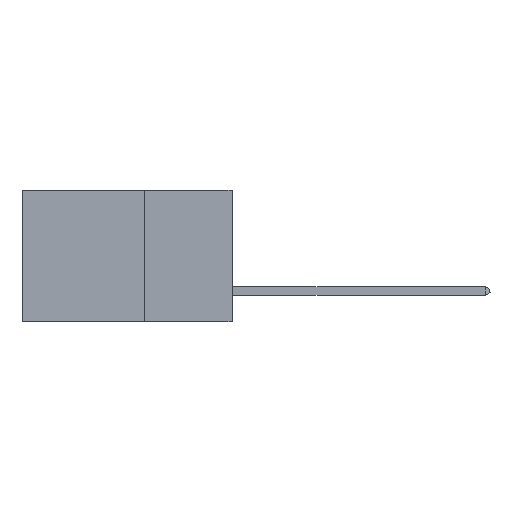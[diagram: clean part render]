
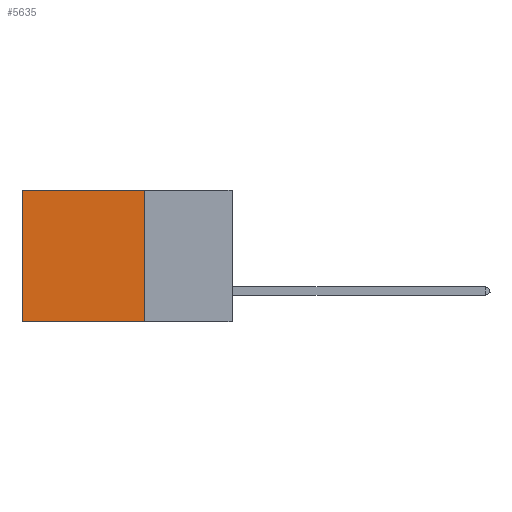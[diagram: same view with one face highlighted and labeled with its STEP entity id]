
A CAD part, left-side view. The second image highlights one B-rep face of the part: STEP entity #5635.
In plain terms, the highlighted planar face has unit normal (-1, 0, 0).
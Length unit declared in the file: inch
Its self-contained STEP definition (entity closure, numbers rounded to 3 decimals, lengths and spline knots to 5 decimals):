
#220 = CARTESIAN_POINT ( 'NONE',  ( 0.2875, 0.25, -0.375 ) ) ;
#1870 = ORIENTED_EDGE ( 'NONE', *, *, #9336, .T. ) ;
#2550 = VECTOR ( 'NONE', #4177, 39.37008 ) ;
#3336 = CARTESIAN_POINT ( 'NONE',  ( 0.2875, 0.6, -0.375 ) ) ;
#4177 = DIRECTION ( 'NONE',  ( 0., 1., 0. ) ) ;
#4750 = VECTOR ( 'NONE', #9437, 39.37008 ) ;
#4900 = LINE ( 'NONE', #13438, #2550 ) ;
#4920 = VECTOR ( 'NONE', #13117, 39.37008 ) ;
#5073 = VERTEX_POINT ( 'NONE', #14737 ) ;
#5245 = PLANE ( 'NONE',  #12274 ) ;
#5388 = EDGE_CURVE ( 'NONE', #11616, #7724, #6596, .T. ) ;
#5635 = ADVANCED_FACE ( 'NONE', ( #8237 ), #5245, .F. ) ;
#6083 = EDGE_CURVE ( 'NONE', #7082, #11616, #10578, .T. ) ;
#6199 = LINE ( 'NONE', #3336, #14768 ) ;
#6369 = DIRECTION ( 'NONE',  ( 0., 0., -1. ) ) ;
#6430 = CARTESIAN_POINT ( 'NONE',  ( 0.2875, 0.6, -0.375 ) ) ;
#6468 = CARTESIAN_POINT ( 'NONE',  ( 0.2875, 0.25, -0.375 ) ) ;
#6596 = LINE ( 'NONE', #9387, #4750 ) ;
#7082 = VERTEX_POINT ( 'NONE', #8293 ) ;
#7724 = VERTEX_POINT ( 'NONE', #6430 ) ;
#8237 = FACE_OUTER_BOUND ( 'NONE', #10676, .T. ) ;
#8293 = CARTESIAN_POINT ( 'NONE',  ( 0.2875, 0.25, 0. ) ) ;
#8301 = CARTESIAN_POINT ( 'NONE',  ( 0.2875, 0.25, -0.375 ) ) ;
#9336 = EDGE_CURVE ( 'NONE', #5073, #7724, #6199, .T. ) ;
#9387 = CARTESIAN_POINT ( 'NONE',  ( 0.2875, 0.25, -0.375 ) ) ;
#9437 = DIRECTION ( 'NONE',  ( 0., 1., 0. ) ) ;
#9484 = ORIENTED_EDGE ( 'NONE', *, *, #6083, .F. ) ;
#10578 = LINE ( 'NONE', #8301, #4920 ) ;
#10589 = EDGE_CURVE ( 'NONE', #7082, #5073, #4900, .T. ) ;
#10676 = EDGE_LOOP ( 'NONE', ( #1870, #13698, #9484, #11854 ) ) ;
#11616 = VERTEX_POINT ( 'NONE', #220 ) ;
#11854 = ORIENTED_EDGE ( 'NONE', *, *, #10589, .T. ) ;
#12274 = AXIS2_PLACEMENT_3D ( 'NONE', #6468, #13379, #6369 ) ;
#12392 = DIRECTION ( 'NONE',  ( 0., 0., -1. ) ) ;
#13117 = DIRECTION ( 'NONE',  ( 0., 0., -1. ) ) ;
#13379 = DIRECTION ( 'NONE',  ( 1., 0., 0. ) ) ;
#13438 = CARTESIAN_POINT ( 'NONE',  ( 0.2875, 0.25, 0. ) ) ;
#13698 = ORIENTED_EDGE ( 'NONE', *, *, #5388, .F. ) ;
#14737 = CARTESIAN_POINT ( 'NONE',  ( 0.2875, 0.6, 0. ) ) ;
#14768 = VECTOR ( 'NONE', #12392, 39.37008 ) ;
